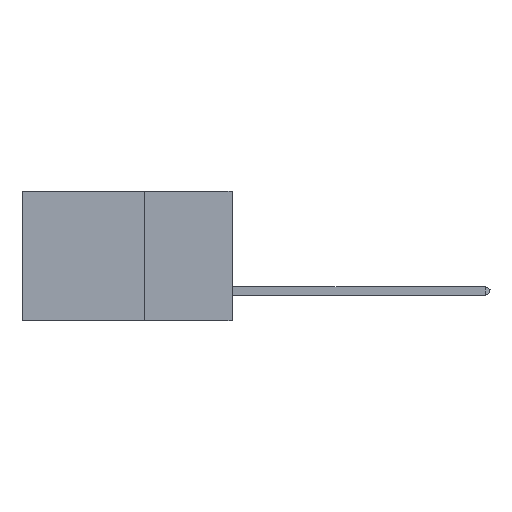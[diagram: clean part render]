
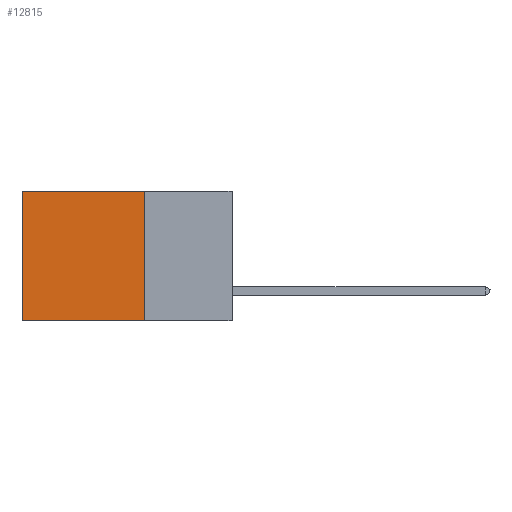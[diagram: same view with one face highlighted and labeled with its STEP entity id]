
A CAD part, left-side view. The second image highlights one B-rep face of the part: STEP entity #12815.
In plain terms, the highlighted planar face has unit normal (-1, 0, 0).
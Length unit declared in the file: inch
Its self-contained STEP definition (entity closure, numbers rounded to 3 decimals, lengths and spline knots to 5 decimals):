
#558 = VERTEX_POINT ( 'NONE', #27066 ) ;
#689 = LINE ( 'NONE', #17067, #22693 ) ;
#1623 = VECTOR ( 'NONE', #19129, 39.37008 ) ;
#2364 = LINE ( 'NONE', #30975, #21717 ) ;
#2968 = EDGE_CURVE ( 'NONE', #558, #5949, #689, .T. ) ;
#3734 = DIRECTION ( 'NONE',  ( 0., 0., -1. ) ) ;
#4753 = ORIENTED_EDGE ( 'NONE', *, *, #12766, .T. ) ;
#4776 = CARTESIAN_POINT ( 'NONE',  ( 0.2875, 0.25, 0. ) ) ;
#4879 = DIRECTION ( 'NONE',  ( 0., 0., -1. ) ) ;
#5418 = VECTOR ( 'NONE', #12058, 39.37008 ) ;
#5668 = EDGE_LOOP ( 'NONE', ( #14212, #30165, #19046, #4753 ) ) ;
#5949 = VERTEX_POINT ( 'NONE', #8110 ) ;
#6089 = EDGE_CURVE ( 'NONE', #30959, #5949, #2364, .T. ) ;
#7371 = AXIS2_PLACEMENT_3D ( 'NONE', #4776, #28777, #3734 ) ;
#8110 = CARTESIAN_POINT ( 'NONE',  ( 0.2875, 0.6, -0.37 ) ) ;
#8217 = CARTESIAN_POINT ( 'NONE',  ( 0.2875, 0.6, 0. ) ) ;
#9669 = CARTESIAN_POINT ( 'NONE',  ( 0.2875, 0.25, 0. ) ) ;
#11808 = FACE_OUTER_BOUND ( 'NONE', #5668, .T. ) ;
#11936 = DIRECTION ( 'NONE',  ( 0., 1., 0. ) ) ;
#12058 = DIRECTION ( 'NONE',  ( 0., 0., -1. ) ) ;
#12644 = VERTEX_POINT ( 'NONE', #24743 ) ;
#12766 = EDGE_CURVE ( 'NONE', #12644, #30959, #25499, .T. ) ;
#12815 = ADVANCED_FACE ( 'NONE', ( #11808 ), #23630, .F. ) ;
#14212 = ORIENTED_EDGE ( 'NONE', *, *, #6089, .T. ) ;
#17067 = CARTESIAN_POINT ( 'NONE',  ( 0.2875, 0.25, -0.37 ) ) ;
#19046 = ORIENTED_EDGE ( 'NONE', *, *, #24322, .F. ) ;
#19129 = DIRECTION ( 'NONE',  ( 0., 1., 0. ) ) ;
#21717 = VECTOR ( 'NONE', #4879, 39.37008 ) ;
#22693 = VECTOR ( 'NONE', #11936, 39.37008 ) ;
#23630 = PLANE ( 'NONE',  #7371 ) ;
#24322 = EDGE_CURVE ( 'NONE', #12644, #558, #26268, .T. ) ;
#24743 = CARTESIAN_POINT ( 'NONE',  ( 0.2875, 0.25, 0. ) ) ;
#25499 = LINE ( 'NONE', #28982, #1623 ) ;
#26268 = LINE ( 'NONE', #9669, #5418 ) ;
#27066 = CARTESIAN_POINT ( 'NONE',  ( 0.2875, 0.25, -0.37 ) ) ;
#28777 = DIRECTION ( 'NONE',  ( 1., 0., 0. ) ) ;
#28982 = CARTESIAN_POINT ( 'NONE',  ( 0.2875, 0.25, 0. ) ) ;
#30165 = ORIENTED_EDGE ( 'NONE', *, *, #2968, .F. ) ;
#30959 = VERTEX_POINT ( 'NONE', #8217 ) ;
#30975 = CARTESIAN_POINT ( 'NONE',  ( 0.2875, 0.6, 0. ) ) ;
